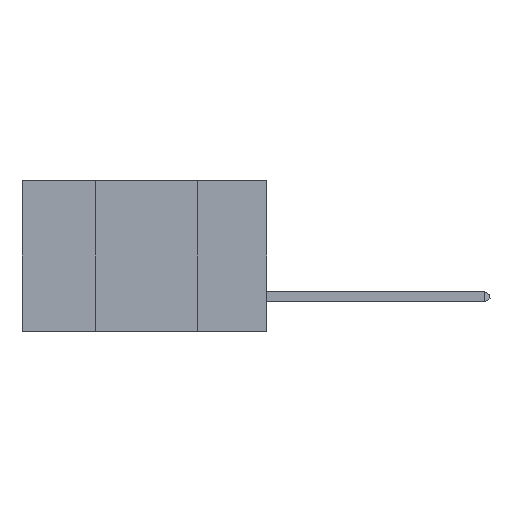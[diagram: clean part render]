
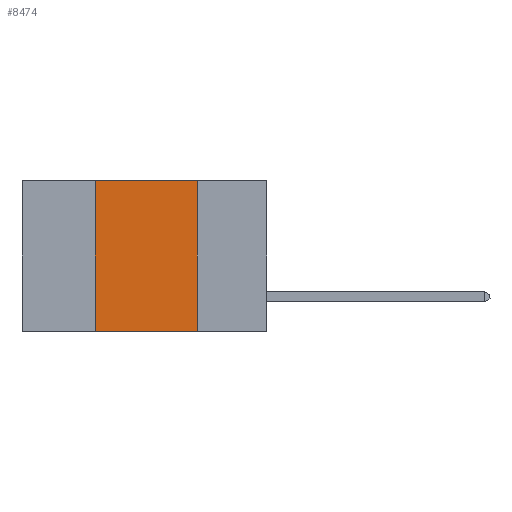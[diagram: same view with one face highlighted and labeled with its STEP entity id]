
A CAD part, left-side view. The second image highlights one B-rep face of the part: STEP entity #8474.
In plain terms, the highlighted planar face has unit normal (-1, 0, 0).
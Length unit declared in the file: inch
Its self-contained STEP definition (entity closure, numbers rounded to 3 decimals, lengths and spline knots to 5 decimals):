
#380 = DIRECTION ( 'NONE',  ( 0., 0., -1. ) ) ;
#597 = VERTEX_POINT ( 'NONE', #12583 ) ;
#2243 = ORIENTED_EDGE ( 'NONE', *, *, #17877, .F. ) ;
#5286 = EDGE_CURVE ( 'NONE', #18427, #597, #8177, .T. ) ;
#6467 = EDGE_CURVE ( 'NONE', #16103, #597, #19957, .T. ) ;
#6845 = CARTESIAN_POINT ( 'NONE',  ( 0., 0.6, -0.37 ) ) ;
#7246 = PLANE ( 'NONE',  #8003 ) ;
#8003 = AXIS2_PLACEMENT_3D ( 'NONE', #16466, #20039, #9107 ) ;
#8177 = LINE ( 'NONE', #22288, #23247 ) ;
#8474 = ADVANCED_FACE ( 'NONE', ( #13987 ), #7246, .F. ) ;
#8711 = DIRECTION ( 'NONE',  ( 0., -1., 0. ) ) ;
#9107 = DIRECTION ( 'NONE',  ( 0., 0., -1. ) ) ;
#9182 = DIRECTION ( 'NONE',  ( 0., 0., 1. ) ) ;
#9976 = EDGE_LOOP ( 'NONE', ( #18116, #14437, #2243, #11749 ) ) ;
#10177 = VECTOR ( 'NONE', #20813, 39.37008 ) ;
#11749 = ORIENTED_EDGE ( 'NONE', *, *, #6467, .T. ) ;
#12583 = CARTESIAN_POINT ( 'NONE',  ( 0., 0.17, -0.37 ) ) ;
#12849 = CARTESIAN_POINT ( 'NONE',  ( 0., 0.42, 0. ) ) ;
#13339 = CARTESIAN_POINT ( 'NONE',  ( 0., 0.42, -0.37 ) ) ;
#13584 = CARTESIAN_POINT ( 'NONE',  ( 0., 0.6, 0. ) ) ;
#13987 = FACE_OUTER_BOUND ( 'NONE', #9976, .T. ) ;
#14437 = ORIENTED_EDGE ( 'NONE', *, *, #20164, .F. ) ;
#15118 = LINE ( 'NONE', #13584, #10177 ) ;
#15769 = VECTOR ( 'NONE', #9182, 39.37008 ) ;
#16103 = VERTEX_POINT ( 'NONE', #13339 ) ;
#16342 = LINE ( 'NONE', #12849, #15769 ) ;
#16360 = CARTESIAN_POINT ( 'NONE',  ( 0., 0.42, 0. ) ) ;
#16466 = CARTESIAN_POINT ( 'NONE',  ( 0., 0.6, 0. ) ) ;
#17877 = EDGE_CURVE ( 'NONE', #16103, #21727, #16342, .T. ) ;
#18116 = ORIENTED_EDGE ( 'NONE', *, *, #5286, .F. ) ;
#18427 = VERTEX_POINT ( 'NONE', #21359 ) ;
#19395 = VECTOR ( 'NONE', #8711, 39.37008 ) ;
#19957 = LINE ( 'NONE', #6845, #19395 ) ;
#20039 = DIRECTION ( 'NONE',  ( 1., 0., 0. ) ) ;
#20164 = EDGE_CURVE ( 'NONE', #21727, #18427, #15118, .T. ) ;
#20813 = DIRECTION ( 'NONE',  ( 0., -1., 0. ) ) ;
#21359 = CARTESIAN_POINT ( 'NONE',  ( 0., 0.17, 0. ) ) ;
#21727 = VERTEX_POINT ( 'NONE', #16360 ) ;
#22288 = CARTESIAN_POINT ( 'NONE',  ( 0., 0.17, 0. ) ) ;
#23247 = VECTOR ( 'NONE', #380, 39.37008 ) ;
